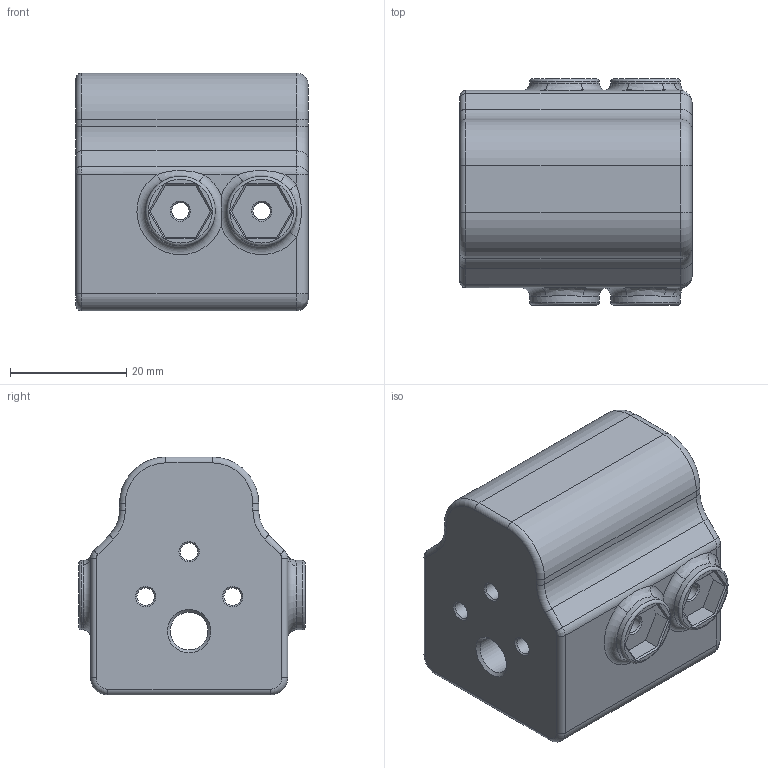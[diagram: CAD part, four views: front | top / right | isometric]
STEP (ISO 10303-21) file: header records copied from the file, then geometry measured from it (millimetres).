
FILE_DESCRIPTION(/* description */ (''),/* implementation_level */ '2;1');
FILE_NAME(/* name */ 'Brace Adapter.step',/* time_stamp */ '2019-04-30T10:08:27-05:00',/* author */ (''),/* organization */ (''),/* preprocessor_version */ 'ST-DEVELOPER v18',/* originating_system */ 'Autodesk Translation Framework v8.2.0.1029',/* authorisation */ '');
FILE_SCHEMA (('AUTOMOTIVE_DESIGN { 1 0 10303 214 3 1 1 }'));
Length unit declared in the file: millimetre
Products named in the file (1): Brace Adapter
Bounding box: 40 x 39 x 41 mm (x, y, z)
Volume: 31534.5 mm3; surface area: 11315.6 mm2
Topology: 1 solids, 1 shells, 159 faces, 385 edges, 231 vertices
Faces by surface type: plane 50, cylinder 42, torus 25, bspline 23, cone 17, sphere 2
Full cylindrical faces by diameter (mm): 3 x7, 6.5 x1, 10 x5, 12 x4, 26 x1
Entity records: 6864 total; most frequent: CARTESIAN_POINT 3086, DIRECTION 811, ORIENTED_EDGE 770, EDGE_CURVE 385, AXIS2_PLACEMENT_3D 329, VERTEX_POINT 231, CIRCLE 189, EDGE_LOOP 178
